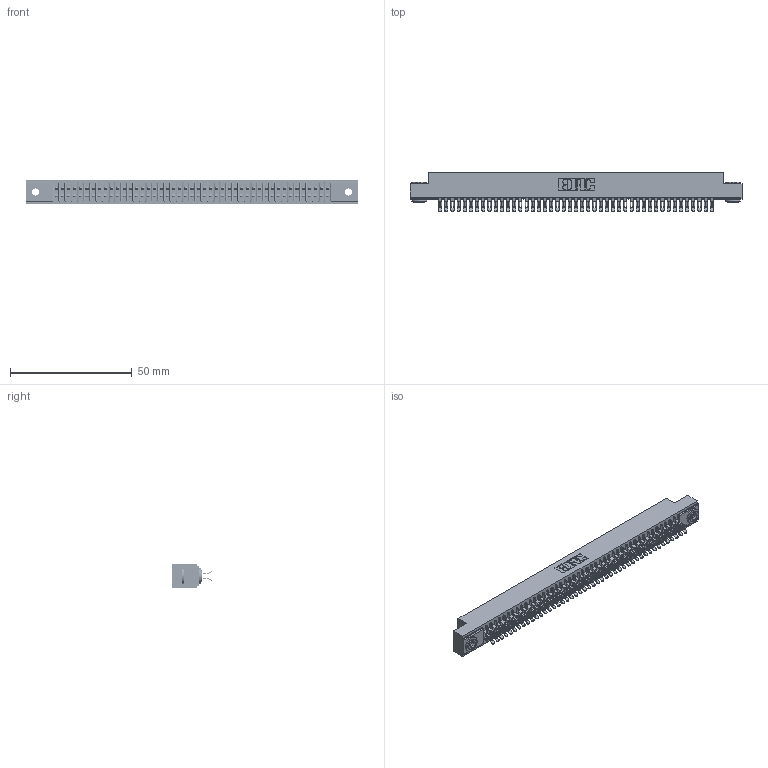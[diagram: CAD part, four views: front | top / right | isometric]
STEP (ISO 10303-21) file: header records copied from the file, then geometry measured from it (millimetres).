
FILE_DESCRIPTION (( 'STEP AP203' ), '1' );
FILE_NAME ('341-090-555-203.STEP', '2018-08-08T00:13:14', ( '' ), ( '' ), 'SwSTEP 2.0', 'SolidWorks 2016', '' );
FILE_SCHEMA (( 'CONFIG_CONTROL_DESIGN' ));
Length unit declared in the file: inch
Products named in the file (4): 341 Part_.156 (3.96) Dia Mounting Holes; 341-292-001_341-292-155; 345-250-002_345-250-002-102; 341-090-555-203
Assembly tree (93 placements, depth 2):
  341-090-555-203
    341 Part_.156 (3.96) Dia Mounting Holes
    341-292-001_341-292-155  x90
    345-250-002_345-250-002-102  x2
Bounding box: 136.53 x 16.31 x 10.16 mm (x, y, z)
Volume: 10200 mm3; surface area: 19179.8 mm2
Topology: 93 solids, 93 shells, 7188 faces, 21443 edges, 13958 vertices
Faces by surface type: plane 3872, cylinder 3128, sphere 92, torus 88, cone 8
Entity records: 55595 total; most frequent: CARTESIAN_POINT 9238, ORIENTED_EDGE 9162, DIRECTION 8969, EDGE_CURVE 4581, LINE 3679, VECTOR 3679, VERTEX_POINT 2898, AXIS2_PLACEMENT_3D 2645
